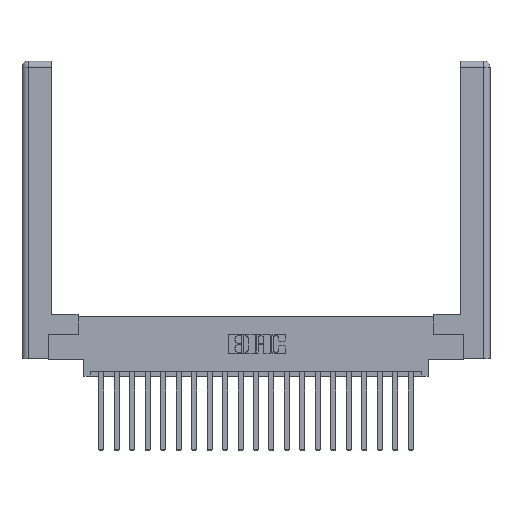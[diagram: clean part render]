
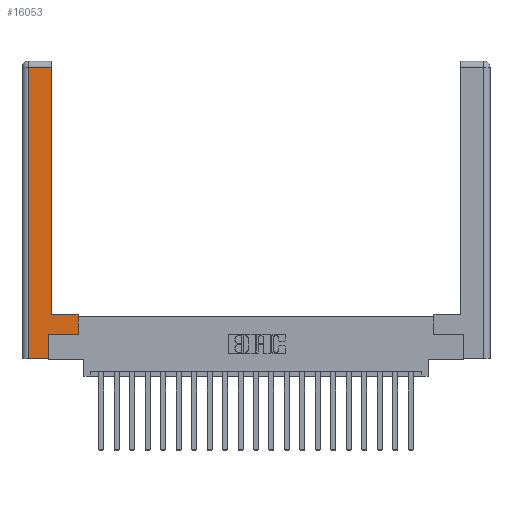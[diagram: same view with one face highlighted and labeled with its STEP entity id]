
A CAD part, top view. The second image highlights one B-rep face of the part: STEP entity #16053.
In plain terms, the highlighted planar face has unit normal (0, 0, 1).
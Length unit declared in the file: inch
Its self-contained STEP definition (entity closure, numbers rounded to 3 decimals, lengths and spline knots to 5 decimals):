
#1025 = EDGE_LOOP ( 'NONE', ( #2402, #13679, #15773, #5606, #17367, #6752, #7089, #11902 ) ) ;
#1282 = EDGE_CURVE ( 'NONE', #5323, #15098, #19819, .T. ) ;
#1612 = VERTEX_POINT ( 'NONE', #16318 ) ;
#1799 = VECTOR ( 'NONE', #15340, 39.37008 ) ;
#2018 = VERTEX_POINT ( 'NONE', #14607 ) ;
#2347 = EDGE_CURVE ( 'NONE', #16727, #2018, #8797, .T. ) ;
#2402 = ORIENTED_EDGE ( 'NONE', *, *, #1282, .T. ) ;
#2989 = EDGE_CURVE ( 'NONE', #15098, #16727, #3352, .T. ) ;
#3352 = LINE ( 'NONE', #15679, #21035 ) ;
#3377 = VECTOR ( 'NONE', #10104, 39.37008 ) ;
#3779 = CARTESIAN_POINT ( 'NONE',  ( 0.295, 0.45, 0. ) ) ;
#4169 = CARTESIAN_POINT ( 'NONE',  ( 0.265, 0., 0. ) ) ;
#4409 = VECTOR ( 'NONE', #17189, 39.37008 ) ;
#4685 = LINE ( 'NONE', #3779, #4409 ) ;
#5323 = VERTEX_POINT ( 'NONE', #17099 ) ;
#5606 = ORIENTED_EDGE ( 'NONE', *, *, #19965, .T. ) ;
#5615 = CARTESIAN_POINT ( 'NONE',  ( 0.0615, 2.94, 0. ) ) ;
#6161 = CARTESIAN_POINT ( 'NONE',  ( 0.565, 0.45, 0. ) ) ;
#6752 = ORIENTED_EDGE ( 'NONE', *, *, #6878, .T. ) ;
#6767 = DIRECTION ( 'NONE',  ( -1., 0., 0. ) ) ;
#6878 = EDGE_CURVE ( 'NONE', #1612, #7124, #9923, .T. ) ;
#7089 = ORIENTED_EDGE ( 'NONE', *, *, #16616, .T. ) ;
#7124 = VERTEX_POINT ( 'NONE', #11795 ) ;
#7265 = LINE ( 'NONE', #17571, #20080 ) ;
#7421 = CARTESIAN_POINT ( 'NONE',  ( 0.0615, 0., 0. ) ) ;
#8481 = CARTESIAN_POINT ( 'NONE',  ( 0., 0., 0. ) ) ;
#8797 = LINE ( 'NONE', #7421, #16954 ) ;
#8834 = VECTOR ( 'NONE', #17017, 39.37008 ) ;
#9476 = CARTESIAN_POINT ( 'NONE',  ( 0.565, 0.245, 0. ) ) ;
#9923 = LINE ( 'NONE', #9476, #8834 ) ;
#10034 = CARTESIAN_POINT ( 'NONE',  ( 0.565, 0.45, 0. ) ) ;
#10104 = DIRECTION ( 'NONE',  ( 0., 1., 0. ) ) ;
#10110 = DIRECTION ( 'NONE',  ( 0., 0., -1. ) ) ;
#10610 = DIRECTION ( 'NONE',  ( 0., 1., 0. ) ) ;
#11795 = CARTESIAN_POINT ( 'NONE',  ( 0.565, 0.245, 0. ) ) ;
#11902 = ORIENTED_EDGE ( 'NONE', *, *, #21126, .T. ) ;
#12249 = EDGE_CURVE ( 'NONE', #21309, #1612, #13855, .T. ) ;
#12256 = AXIS2_PLACEMENT_3D ( 'NONE', #8481, #10110, #6767 ) ;
#12723 = VERTEX_POINT ( 'NONE', #6161 ) ;
#13679 = ORIENTED_EDGE ( 'NONE', *, *, #2989, .T. ) ;
#13855 = LINE ( 'NONE', #19005, #17785 ) ;
#14297 = LINE ( 'NONE', #10034, #3377 ) ;
#14607 = CARTESIAN_POINT ( 'NONE',  ( 0.0615, 0., 0. ) ) ;
#15098 = VERTEX_POINT ( 'NONE', #19940 ) ;
#15340 = DIRECTION ( 'NONE',  ( 0., 1., 0. ) ) ;
#15679 = CARTESIAN_POINT ( 'NONE',  ( 0.0615, 2.94, 0. ) ) ;
#15773 = ORIENTED_EDGE ( 'NONE', *, *, #2347, .T. ) ;
#15960 = DIRECTION ( 'NONE',  ( -1., 0., 0. ) ) ;
#16053 = ADVANCED_FACE ( 'NONE', ( #16980 ), #16989, .F. ) ;
#16318 = CARTESIAN_POINT ( 'NONE',  ( 0.265, 0.245, 0. ) ) ;
#16616 = EDGE_CURVE ( 'NONE', #7124, #12723, #14297, .T. ) ;
#16727 = VERTEX_POINT ( 'NONE', #5615 ) ;
#16954 = VECTOR ( 'NONE', #21049, 39.37008 ) ;
#16980 = FACE_OUTER_BOUND ( 'NONE', #1025, .T. ) ;
#16989 = PLANE ( 'NONE',  #12256 ) ;
#17017 = DIRECTION ( 'NONE',  ( 1., 0., 0. ) ) ;
#17099 = CARTESIAN_POINT ( 'NONE',  ( 0.295, 0.45, 0. ) ) ;
#17189 = DIRECTION ( 'NONE',  ( -1., 0., 0. ) ) ;
#17367 = ORIENTED_EDGE ( 'NONE', *, *, #12249, .T. ) ;
#17571 = CARTESIAN_POINT ( 'NONE',  ( 0.265, 0., 0. ) ) ;
#17785 = VECTOR ( 'NONE', #10610, 39.37008 ) ;
#18533 = CARTESIAN_POINT ( 'NONE',  ( 0.295, 3., 0. ) ) ;
#19005 = CARTESIAN_POINT ( 'NONE',  ( 0.265, 0.245, 0. ) ) ;
#19295 = DIRECTION ( 'NONE',  ( 1., 0., 0. ) ) ;
#19819 = LINE ( 'NONE', #18533, #1799 ) ;
#19940 = CARTESIAN_POINT ( 'NONE',  ( 0.295, 2.94, 0. ) ) ;
#19965 = EDGE_CURVE ( 'NONE', #2018, #21309, #7265, .T. ) ;
#20080 = VECTOR ( 'NONE', #19295, 39.37008 ) ;
#21035 = VECTOR ( 'NONE', #15960, 39.37008 ) ;
#21049 = DIRECTION ( 'NONE',  ( 0., -1., 0. ) ) ;
#21126 = EDGE_CURVE ( 'NONE', #12723, #5323, #4685, .T. ) ;
#21309 = VERTEX_POINT ( 'NONE', #4169 ) ;
